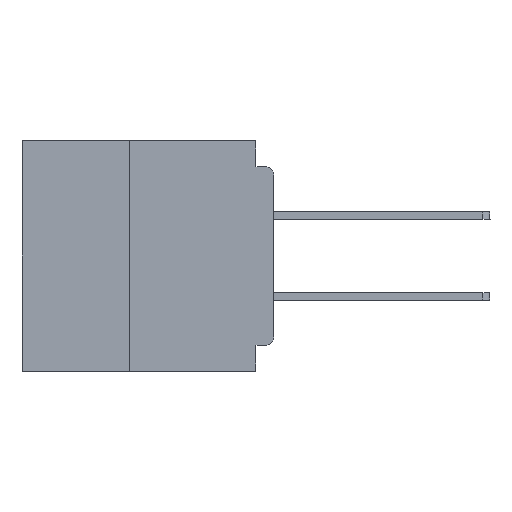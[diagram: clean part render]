
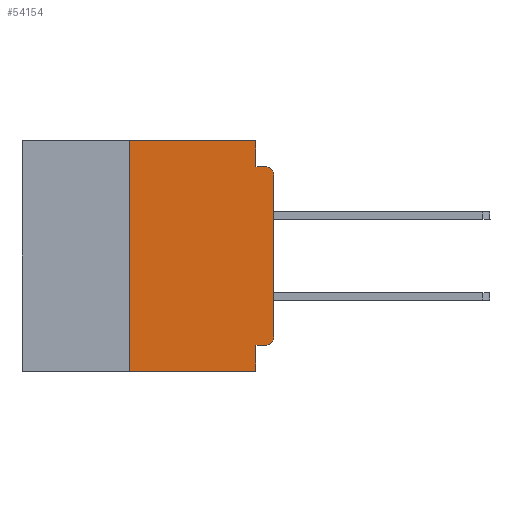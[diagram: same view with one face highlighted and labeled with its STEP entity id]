
A CAD part, left-side view. The second image highlights one B-rep face of the part: STEP entity #54154.
In plain terms, the highlighted planar face has unit normal (-1, 0, 0).
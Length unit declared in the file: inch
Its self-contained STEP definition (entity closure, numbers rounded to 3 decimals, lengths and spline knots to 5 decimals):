
#1250 = CARTESIAN_POINT ( 'NONE',  ( 0., 0.031, -0.355 ) ) ;
#2470 = EDGE_CURVE ( 'NONE', #59918, #21871, #14757, .T. ) ;
#3630 = VECTOR ( 'NONE', #27994, 39.37008 ) ;
#5142 = PLANE ( 'NONE',  #64386 ) ;
#6218 = ORIENTED_EDGE ( 'NONE', *, *, #6248, .T. ) ;
#6248 = EDGE_CURVE ( 'NONE', #43769, #13845, #17484, .T. ) ;
#6825 = VECTOR ( 'NONE', #48463, 39.37008 ) ;
#8060 = CARTESIAN_POINT ( 'NONE',  ( 0., 0.437, -0.4 ) ) ;
#10895 = ORIENTED_EDGE ( 'NONE', *, *, #30855, .F. ) ;
#11499 = CARTESIAN_POINT ( 'NONE',  ( 0., 0.015, -0.34 ) ) ;
#11551 = AXIS2_PLACEMENT_3D ( 'NONE', #11499, #46588, #16578 ) ;
#11679 = CARTESIAN_POINT ( 'NONE',  ( 0., 0.031, -0.045 ) ) ;
#11941 = ORIENTED_EDGE ( 'NONE', *, *, #55213, .F. ) ;
#13845 = VERTEX_POINT ( 'NONE', #51197 ) ;
#14154 = ORIENTED_EDGE ( 'NONE', *, *, #2470, .F. ) ;
#14757 = LINE ( 'NONE', #31512, #54644 ) ;
#15502 = EDGE_LOOP ( 'NONE', ( #6218, #37984, #10895, #14154, #41949, #11941, #42840, #34992, #49512, #55660 ) ) ;
#15985 = DIRECTION ( 'NONE',  ( -1., 0., 0. ) ) ;
#16498 = VERTEX_POINT ( 'NONE', #58595 ) ;
#16578 = DIRECTION ( 'NONE',  ( 0., 0., -1. ) ) ;
#17484 = LINE ( 'NONE', #39922, #55759 ) ;
#18380 = VECTOR ( 'NONE', #43215, 39.37008 ) ;
#18546 = DIRECTION ( 'NONE',  ( 0., -1., 0. ) ) ;
#20395 = DIRECTION ( 'NONE',  ( 1., 0., 0. ) ) ;
#20710 = EDGE_CURVE ( 'NONE', #31087, #45827, #37767, .T. ) ;
#21016 = CARTESIAN_POINT ( 'NONE',  ( 0., 0., -0.34 ) ) ;
#21871 = VERTEX_POINT ( 'NONE', #11679 ) ;
#22394 = CARTESIAN_POINT ( 'NONE',  ( 0., 0., -0.355 ) ) ;
#22983 = EDGE_CURVE ( 'NONE', #13845, #48845, #24975, .T. ) ;
#24975 = CIRCLE ( 'NONE', #39995, 0.015 ) ;
#26048 = VERTEX_POINT ( 'NONE', #63031 ) ;
#27994 = DIRECTION ( 'NONE',  ( 0., 0., -1. ) ) ;
#30454 = LINE ( 'NONE', #38144, #3630 ) ;
#30855 = EDGE_CURVE ( 'NONE', #21871, #48845, #48552, .T. ) ;
#31087 = VERTEX_POINT ( 'NONE', #62533 ) ;
#31303 = DIRECTION ( 'NONE',  ( 0., 0., -1. ) ) ;
#31512 = CARTESIAN_POINT ( 'NONE',  ( 0., 0.031, 0. ) ) ;
#31712 = LINE ( 'NONE', #8060, #18380 ) ;
#34992 = ORIENTED_EDGE ( 'NONE', *, *, #35394, .F. ) ;
#35343 = CARTESIAN_POINT ( 'NONE',  ( 0., 0.437, 0. ) ) ;
#35394 = EDGE_CURVE ( 'NONE', #45827, #35818, #30454, .T. ) ;
#35818 = VERTEX_POINT ( 'NONE', #46526 ) ;
#37427 = CARTESIAN_POINT ( 'NONE',  ( 0., 0.031, 0. ) ) ;
#37503 = CARTESIAN_POINT ( 'NONE',  ( 0., 0.015, -0.045 ) ) ;
#37767 = LINE ( 'NONE', #22394, #62527 ) ;
#37984 = ORIENTED_EDGE ( 'NONE', *, *, #22983, .T. ) ;
#38144 = CARTESIAN_POINT ( 'NONE',  ( 0., 0.031, -0.4 ) ) ;
#39440 = EDGE_CURVE ( 'NONE', #16498, #59918, #57593, .T. ) ;
#39922 = CARTESIAN_POINT ( 'NONE',  ( 0., 0., 0. ) ) ;
#39995 = AXIS2_PLACEMENT_3D ( 'NONE', #46006, #15985, #50988 ) ;
#40127 = DIRECTION ( 'NONE',  ( 0., 0., 1. ) ) ;
#40936 = CARTESIAN_POINT ( 'NONE',  ( 0., 0., -0.045 ) ) ;
#41358 = VECTOR ( 'NONE', #18546, 39.37008 ) ;
#41522 = EDGE_CURVE ( 'NONE', #26048, #35818, #31712, .T. ) ;
#41617 = FACE_OUTER_BOUND ( 'NONE', #15502, .T. ) ;
#41949 = ORIENTED_EDGE ( 'NONE', *, *, #39440, .F. ) ;
#42840 = ORIENTED_EDGE ( 'NONE', *, *, #41522, .T. ) ;
#43215 = DIRECTION ( 'NONE',  ( 0., -1., 0. ) ) ;
#43769 = VERTEX_POINT ( 'NONE', #21016 ) ;
#45827 = VERTEX_POINT ( 'NONE', #1250 ) ;
#46006 = CARTESIAN_POINT ( 'NONE',  ( 0., 0.015, -0.06 ) ) ;
#46526 = CARTESIAN_POINT ( 'NONE',  ( 0., 0.031, -0.4 ) ) ;
#46588 = DIRECTION ( 'NONE',  ( -1., 0., 0. ) ) ;
#48463 = DIRECTION ( 'NONE',  ( 0., 0., 1. ) ) ;
#48498 = CARTESIAN_POINT ( 'NONE',  ( 0., 0.437, 0. ) ) ;
#48552 = LINE ( 'NONE', #40936, #61694 ) ;
#48845 = VERTEX_POINT ( 'NONE', #37503 ) ;
#49512 = ORIENTED_EDGE ( 'NONE', *, *, #20710, .F. ) ;
#50988 = DIRECTION ( 'NONE',  ( 0., 0., -1. ) ) ;
#51197 = CARTESIAN_POINT ( 'NONE',  ( 0., 0., -0.06 ) ) ;
#54154 = ADVANCED_FACE ( 'NONE', ( #41617 ), #5142, .F. ) ;
#54644 = VECTOR ( 'NONE', #31303, 39.37008 ) ;
#55213 = EDGE_CURVE ( 'NONE', #26048, #16498, #58483, .T. ) ;
#55307 = DIRECTION ( 'NONE',  ( 0., 0., -1. ) ) ;
#55660 = ORIENTED_EDGE ( 'NONE', *, *, #62549, .T. ) ;
#55759 = VECTOR ( 'NONE', #40127, 39.37008 ) ;
#57262 = DIRECTION ( 'NONE',  ( 0., 1., 0. ) ) ;
#57593 = LINE ( 'NONE', #48498, #41358 ) ;
#58352 = CIRCLE ( 'NONE', #11551, 0.015 ) ;
#58390 = CARTESIAN_POINT ( 'NONE',  ( 0., 0.25, -0.4 ) ) ;
#58483 = LINE ( 'NONE', #58390, #6825 ) ;
#58595 = CARTESIAN_POINT ( 'NONE',  ( 0., 0.25, 0. ) ) ;
#59918 = VERTEX_POINT ( 'NONE', #37427 ) ;
#60848 = DIRECTION ( 'NONE',  ( 0., -1., 0. ) ) ;
#61694 = VECTOR ( 'NONE', #60848, 39.37008 ) ;
#62527 = VECTOR ( 'NONE', #57262, 39.37008 ) ;
#62533 = CARTESIAN_POINT ( 'NONE',  ( 0., 0.015, -0.355 ) ) ;
#62549 = EDGE_CURVE ( 'NONE', #31087, #43769, #58352, .T. ) ;
#63031 = CARTESIAN_POINT ( 'NONE',  ( 0., 0.25, -0.4 ) ) ;
#64386 = AXIS2_PLACEMENT_3D ( 'NONE', #35343, #20395, #55307 ) ;
